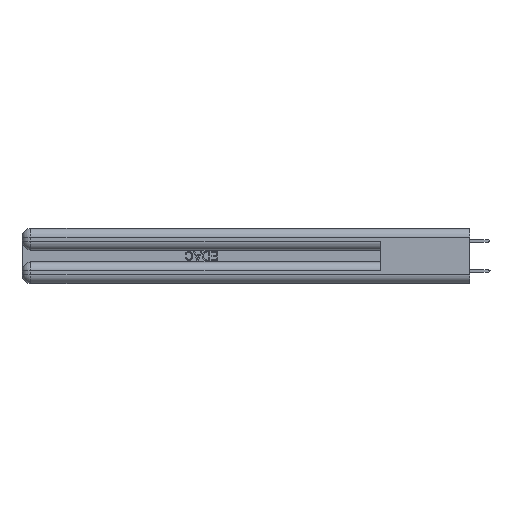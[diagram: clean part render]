
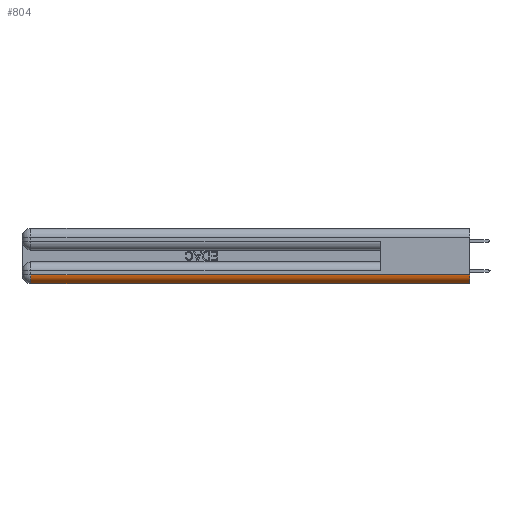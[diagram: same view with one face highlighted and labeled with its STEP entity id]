
A CAD part, left-side view. The second image highlights one B-rep face of the part: STEP entity #804.
In plain terms, the highlighted cylindrical face has radius 1.524 mm (diameter 3.048 mm), a partial arc.
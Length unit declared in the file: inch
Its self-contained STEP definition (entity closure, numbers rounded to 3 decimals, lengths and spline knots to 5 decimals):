
#514 = CARTESIAN_POINT ( 'NONE',  ( 0., 0., 0.06 ) ) ;
#786 = LINE ( 'NONE', #13986, #28475 ) ;
#804 = ADVANCED_FACE ( 'NONE', ( #37779 ), #8992, .T. ) ;
#1840 = AXIS2_PLACEMENT_3D ( 'NONE', #33269, #16686, #10609 ) ;
#3766 = AXIS2_PLACEMENT_3D ( 'NONE', #36737, #32750, #23686 ) ;
#6412 = CARTESIAN_POINT ( 'NONE',  ( 0., 2.94, 0.06 ) ) ;
#8573 = DIRECTION ( 'NONE',  ( 0., 0., 1. ) ) ;
#8992 = CYLINDRICAL_SURFACE ( 'NONE', #23430, 0.06 ) ;
#10609 = DIRECTION ( 'NONE',  ( 0., 0., 1. ) ) ;
#11201 = EDGE_CURVE ( 'NONE', #32393, #25809, #786, .T. ) ;
#11575 = CARTESIAN_POINT ( 'NONE',  ( 0., 0., 0.06 ) ) ;
#13986 = CARTESIAN_POINT ( 'NONE',  ( 0.06, 3., 0. ) ) ;
#14392 = EDGE_CURVE ( 'NONE', #25809, #16398, #17150, .T. ) ;
#14620 = CARTESIAN_POINT ( 'NONE',  ( 0.06, 0., 0.06 ) ) ;
#15599 = VECTOR ( 'NONE', #20994, 39.37008 ) ;
#16398 = VERTEX_POINT ( 'NONE', #6412 ) ;
#16488 = EDGE_CURVE ( 'NONE', #31464, #32393, #19252, .T. ) ;
#16686 = DIRECTION ( 'NONE',  ( 0., -1., 0. ) ) ;
#17150 = CIRCLE ( 'NONE', #3766, 0.06 ) ;
#19252 = CIRCLE ( 'NONE', #1840, 0.06 ) ;
#19701 = CARTESIAN_POINT ( 'NONE',  ( 0.06, 0., 0. ) ) ;
#20994 = DIRECTION ( 'NONE',  ( 0., -1., 0. ) ) ;
#21971 = DIRECTION ( 'NONE',  ( 0., 1., 0. ) ) ;
#22467 = CARTESIAN_POINT ( 'NONE',  ( 0.06, 2.94, 0. ) ) ;
#23430 = AXIS2_PLACEMENT_3D ( 'NONE', #14620, #21971, #8573 ) ;
#23686 = DIRECTION ( 'NONE',  ( 0., 0., 1. ) ) ;
#24004 = ORIENTED_EDGE ( 'NONE', *, *, #11201, .F. ) ;
#25809 = VERTEX_POINT ( 'NONE', #22467 ) ;
#28475 = VECTOR ( 'NONE', #36484, 39.37008 ) ;
#29196 = ORIENTED_EDGE ( 'NONE', *, *, #14392, .F. ) ;
#29923 = EDGE_LOOP ( 'NONE', ( #39023, #31575, #29196, #24004 ) ) ;
#31464 = VERTEX_POINT ( 'NONE', #514 ) ;
#31575 = ORIENTED_EDGE ( 'NONE', *, *, #35573, .F. ) ;
#32393 = VERTEX_POINT ( 'NONE', #19701 ) ;
#32750 = DIRECTION ( 'NONE',  ( 0., 1., 0. ) ) ;
#33269 = CARTESIAN_POINT ( 'NONE',  ( 0.06, 0., 0.06 ) ) ;
#35573 = EDGE_CURVE ( 'NONE', #16398, #31464, #40371, .T. ) ;
#36484 = DIRECTION ( 'NONE',  ( 0., 1., 0. ) ) ;
#36737 = CARTESIAN_POINT ( 'NONE',  ( 0.06, 2.94, 0.06 ) ) ;
#37779 = FACE_OUTER_BOUND ( 'NONE', #29923, .T. ) ;
#39023 = ORIENTED_EDGE ( 'NONE', *, *, #16488, .F. ) ;
#40371 = LINE ( 'NONE', #11575, #15599 ) ;
